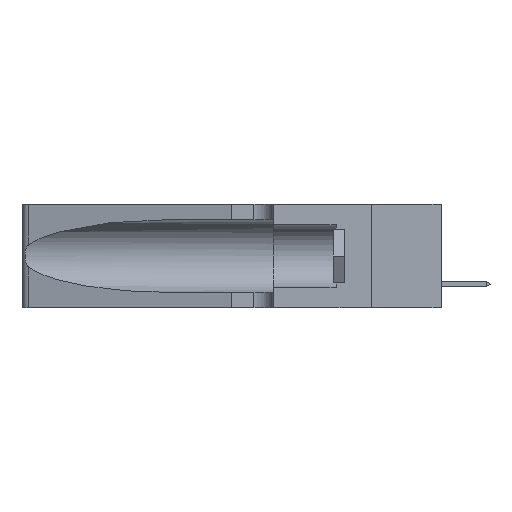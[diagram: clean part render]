
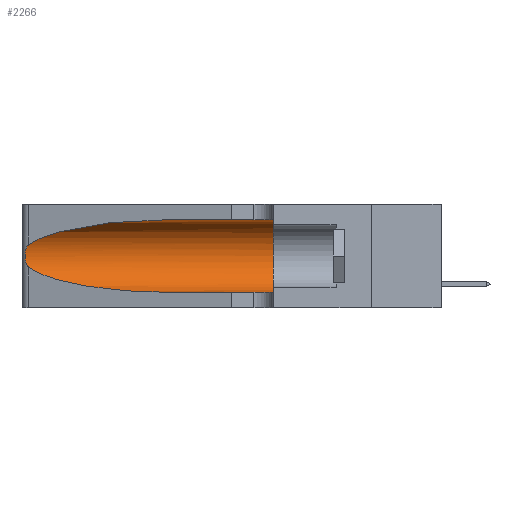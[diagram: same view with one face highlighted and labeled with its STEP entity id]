
A CAD part, left-side view. The second image highlights one B-rep face of the part: STEP entity #2266.
In plain terms, the highlighted cylindrical face has radius 3.308 mm (diameter 6.617 mm), a partial arc.
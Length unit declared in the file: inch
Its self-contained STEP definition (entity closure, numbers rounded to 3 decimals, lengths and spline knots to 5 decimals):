
#80 = CARTESIAN_POINT ( 'NONE',  ( 0.25787, 1.23484, 0.2124 ) ) ;
#410 = CARTESIAN_POINT ( 'NONE',  ( 0.26075, 1.23896, 0.19203 ) ) ;
#644 = EDGE_CURVE ( 'NONE', #14508, #28657, #13195, .T. ) ;
#1528 = ORIENTED_EDGE ( 'NONE', *, *, #18455, .T. ) ;
#1546 =( BOUNDED_CURVE ( )  B_SPLINE_CURVE ( 3, ( #22314, #25697, #30731, #10623 ),
 .UNSPECIFIED., .F., .T. ) 
 B_SPLINE_CURVE_WITH_KNOTS ( ( 4, 4 ),
 ( 1.5708, 2.84003 ),
 .UNSPECIFIED. ) 
 CURVE ( )  GEOMETRIC_REPRESENTATION_ITEM ( )  RATIONAL_B_SPLINE_CURVE ( ( 1., 0.87, 0.87, 1. ) ) 
 REPRESENTATION_ITEM ( '' )  );
#2266 = ADVANCED_FACE ( 'NONE', ( #16334 ), #31337, .F. ) ;
#2320 = CARTESIAN_POINT ( 'NONE',  ( 0.1305, 1.61858, 0.185 ) ) ;
#2387 = CARTESIAN_POINT ( 'NONE',  ( 0.26075, 1.23896, 0.178 ) ) ;
#2605 = CARTESIAN_POINT ( 'NONE',  ( 0.25856, 1.23593, 0.16098 ) ) ;
#4920 = ORIENTED_EDGE ( 'NONE', *, *, #644, .T. ) ;
#4933 = DIRECTION ( 'NONE',  ( 0., -1., 0. ) ) ;
#5107 = CARTESIAN_POINT ( 'NONE',  ( 0.25555, 1.22994, 0.2215 ) ) ;
#5824 = VECTOR ( 'NONE', #21986, 39.37008 ) ;
#6478 = CARTESIAN_POINT ( 'NONE',  ( 0.25487, 1.22718, 0.14631 ) ) ;
#7168 = CARTESIAN_POINT ( 'NONE',  ( 0.25789, 1.23486, 0.15765 ) ) ;
#8253 = CARTESIAN_POINT ( 'NONE',  ( 0.2373, 1.15595, 0.08982 ) ) ;
#10623 = CARTESIAN_POINT ( 'NONE',  ( 0.25487, 1.22718, 0.22369 ) ) ;
#10801 = CARTESIAN_POINT ( 'NONE',  ( 0.18966, 0.96281, 0.05475 ) ) ;
#10974 = LINE ( 'NONE', #20475, #28307 ) ;
#12469 = AXIS2_PLACEMENT_3D ( 'NONE', #2320, #4933, #17558 ) ;
#12540 = CARTESIAN_POINT ( 'NONE',  ( 0.26017, 1.23833, 0.17102 ) ) ;
#13195 =( BOUNDED_CURVE ( )  B_SPLINE_CURVE ( 3, ( #25750, #8253, #10801, #21054 ),
 .UNSPECIFIED., .F., .T. ) 
 B_SPLINE_CURVE_WITH_KNOTS ( ( 4, 4 ),
 ( 3.44316, 4.71239 ),
 .UNSPECIFIED. ) 
 CURVE ( )  GEOMETRIC_REPRESENTATION_ITEM ( )  RATIONAL_B_SPLINE_CURVE ( ( 1., 0.87, 0.87, 1. ) ) 
 REPRESENTATION_ITEM ( '' )  );
#14373 = VERTEX_POINT ( 'NONE', #18552 ) ;
#14508 = VERTEX_POINT ( 'NONE', #6478 ) ;
#15034 = EDGE_CURVE ( 'NONE', #30853, #14373, #10974, .T. ) ;
#15085 = CARTESIAN_POINT ( 'NONE',  ( 0.25639, 1.23184, 0.21858 ) ) ;
#16334 = FACE_OUTER_BOUND ( 'NONE', #22135, .T. ) ;
#17292 = CARTESIAN_POINT ( 'NONE',  ( 0.1305, 1.61858, 0.05475 ) ) ;
#17558 = DIRECTION ( 'NONE',  ( 0., 0., -1. ) ) ;
#18455 = EDGE_CURVE ( 'NONE', #30853, #25927, #1546, .T. ) ;
#18552 = CARTESIAN_POINT ( 'NONE',  ( 0.1305, 0.35, 0.31525 ) ) ;
#19234 = EDGE_CURVE ( 'NONE', #28657, #21471, #29122, .T. ) ;
#19738 = ORIENTED_EDGE ( 'NONE', *, *, #26692, .F. ) ;
#20326 = DIRECTION ( 'NONE',  ( 0., 1., 0. ) ) ;
#20475 = CARTESIAN_POINT ( 'NONE',  ( 0.1305, 1.61858, 0.31525 ) ) ;
#20858 = AXIS2_PLACEMENT_3D ( 'NONE', #24694, #20326, #25325 ) ;
#21054 = CARTESIAN_POINT ( 'NONE',  ( 0.1305, 0.72297, 0.05475 ) ) ;
#21471 = VERTEX_POINT ( 'NONE', #29012 ) ;
#21848 = CARTESIAN_POINT ( 'NONE',  ( 0.1305, 0.72297, 0.31525 ) ) ;
#21986 = DIRECTION ( 'NONE',  ( 0., -1., 0. ) ) ;
#22135 = EDGE_LOOP ( 'NONE', ( #1528, #22234, #4920, #27038, #19738, #27221 ) ) ;
#22234 = ORIENTED_EDGE ( 'NONE', *, *, #26239, .T. ) ;
#22314 = CARTESIAN_POINT ( 'NONE',  ( 0.1305, 0.72297, 0.31525 ) ) ;
#22823 = CARTESIAN_POINT ( 'NONE',  ( 0.25487, 1.22718, 0.14631 ) ) ;
#22926 = CARTESIAN_POINT ( 'NONE',  ( 0.25639, 1.23186, 0.15144 ) ) ;
#24694 = CARTESIAN_POINT ( 'NONE',  ( 0.1305, 0.35, 0.185 ) ) ;
#25042 = CARTESIAN_POINT ( 'NONE',  ( 0.25555, 1.22993, 0.14849 ) ) ;
#25325 = DIRECTION ( 'NONE',  ( 0., 0., 1. ) ) ;
#25584 = CIRCLE ( 'NONE', #20858, 0.13025 ) ;
#25697 = CARTESIAN_POINT ( 'NONE',  ( 0.18966, 0.96281, 0.31525 ) ) ;
#25750 = CARTESIAN_POINT ( 'NONE',  ( 0.25487, 1.22718, 0.14631 ) ) ;
#25927 = VERTEX_POINT ( 'NONE', #29176 ) ;
#26239 = EDGE_CURVE ( 'NONE', #25927, #14508, #28332, .T. ) ;
#26692 = EDGE_CURVE ( 'NONE', #14373, #21471, #25584, .T. ) ;
#27038 = ORIENTED_EDGE ( 'NONE', *, *, #19234, .T. ) ;
#27221 = ORIENTED_EDGE ( 'NONE', *, *, #15034, .F. ) ;
#27569 = CARTESIAN_POINT ( 'NONE',  ( 0.25854, 1.2359, 0.20912 ) ) ;
#27763 = CARTESIAN_POINT ( 'NONE',  ( 0.1305, 0.72297, 0.05475 ) ) ;
#28014 = DIRECTION ( 'NONE',  ( 0., -1., 0. ) ) ;
#28307 = VECTOR ( 'NONE', #28014, 39.37008 ) ;
#28332 = B_SPLINE_CURVE_WITH_KNOTS ( 'NONE', 3,
 ( #30599, #5107, #15085, #80, #27569, #30262, #410, #2387, #12540, #2605, #7168, #22926, #25042, #22823 ),
 .UNSPECIFIED., .F., .F.,
 ( 4, 2, 2, 2, 2, 2, 4 ),
 ( 0., 0.00027, 0.00053, 0.00107, 0.0016, 0.00187, 0.00214 ),
 .UNSPECIFIED. ) ;
#28657 = VERTEX_POINT ( 'NONE', #27763 ) ;
#29012 = CARTESIAN_POINT ( 'NONE',  ( 0.1305, 0.35, 0.05475 ) ) ;
#29122 = LINE ( 'NONE', #17292, #5824 ) ;
#29176 = CARTESIAN_POINT ( 'NONE',  ( 0.25487, 1.22718, 0.22369 ) ) ;
#30262 = CARTESIAN_POINT ( 'NONE',  ( 0.26018, 1.23835, 0.19895 ) ) ;
#30599 = CARTESIAN_POINT ( 'NONE',  ( 0.25487, 1.22718, 0.22369 ) ) ;
#30731 = CARTESIAN_POINT ( 'NONE',  ( 0.2373, 1.15595, 0.28018 ) ) ;
#30853 = VERTEX_POINT ( 'NONE', #21848 ) ;
#31337 = CYLINDRICAL_SURFACE ( 'NONE', #12469, 0.13025 ) ;
